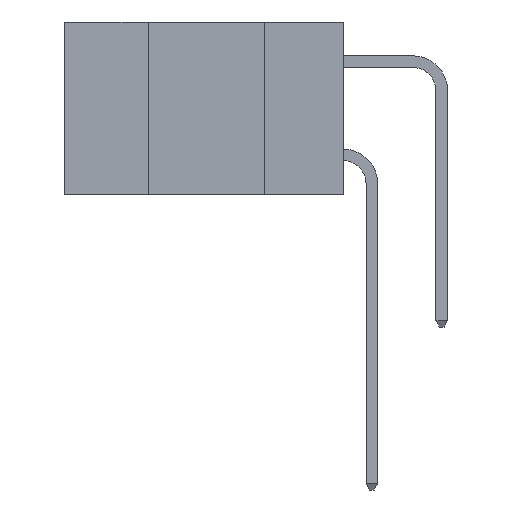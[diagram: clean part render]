
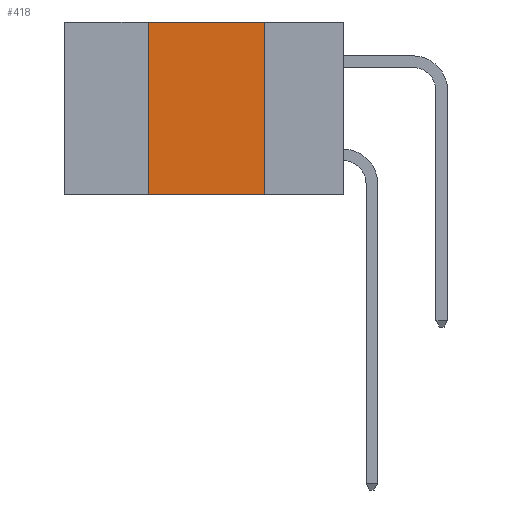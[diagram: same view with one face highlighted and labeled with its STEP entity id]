
A CAD part, left-side view. The second image highlights one B-rep face of the part: STEP entity #418.
In plain terms, the highlighted planar face has unit normal (-1, 0, 0).
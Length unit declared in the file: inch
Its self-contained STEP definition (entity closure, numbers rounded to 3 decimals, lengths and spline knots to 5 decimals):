
#340 = CARTESIAN_POINT ( 'NONE',  ( 0., 0.6, -0.37 ) ) ;
#369 = EDGE_CURVE ( 'NONE', #6488, #3196, #8208, .T. ) ;
#418 = ADVANCED_FACE ( 'NONE', ( #5641 ), #8332, .F. ) ;
#494 = AXIS2_PLACEMENT_3D ( 'NONE', #7348, #6363, #9915 ) ;
#639 = EDGE_CURVE ( 'NONE', #6488, #5417, #9170, .T. ) ;
#745 = DIRECTION ( 'NONE',  ( 0., -1., 0. ) ) ;
#939 = CARTESIAN_POINT ( 'NONE',  ( 0., 0.6, 0. ) ) ;
#1152 = VERTEX_POINT ( 'NONE', #2758 ) ;
#2500 = VECTOR ( 'NONE', #10868, 39.37008 ) ;
#2507 = ORIENTED_EDGE ( 'NONE', *, *, #369, .T. ) ;
#2758 = CARTESIAN_POINT ( 'NONE',  ( 0., 0.17, 0. ) ) ;
#3020 = LINE ( 'NONE', #939, #2500 ) ;
#3196 = VERTEX_POINT ( 'NONE', #7700 ) ;
#3681 = CARTESIAN_POINT ( 'NONE',  ( 0., 0.42, -0.37 ) ) ;
#3735 = DIRECTION ( 'NONE',  ( 0., 0., 1. ) ) ;
#4081 = CARTESIAN_POINT ( 'NONE',  ( 0., 0.42, 0. ) ) ;
#4154 = EDGE_CURVE ( 'NONE', #5417, #1152, #3020, .T. ) ;
#4572 = EDGE_CURVE ( 'NONE', #1152, #3196, #6546, .T. ) ;
#4858 = VECTOR ( 'NONE', #3735, 39.37008 ) ;
#4903 = DIRECTION ( 'NONE',  ( 0., 0., -1. ) ) ;
#5268 = VECTOR ( 'NONE', #745, 39.37008 ) ;
#5321 = ORIENTED_EDGE ( 'NONE', *, *, #4572, .F. ) ;
#5417 = VERTEX_POINT ( 'NONE', #4081 ) ;
#5641 = FACE_OUTER_BOUND ( 'NONE', #7751, .T. ) ;
#6363 = DIRECTION ( 'NONE',  ( 1., 0., 0. ) ) ;
#6488 = VERTEX_POINT ( 'NONE', #10600 ) ;
#6546 = LINE ( 'NONE', #10422, #8708 ) ;
#6943 = ORIENTED_EDGE ( 'NONE', *, *, #4154, .F. ) ;
#7348 = CARTESIAN_POINT ( 'NONE',  ( 0., 0.6, 0. ) ) ;
#7700 = CARTESIAN_POINT ( 'NONE',  ( 0., 0.17, -0.37 ) ) ;
#7751 = EDGE_LOOP ( 'NONE', ( #5321, #6943, #9878, #2507 ) ) ;
#8208 = LINE ( 'NONE', #340, #5268 ) ;
#8332 = PLANE ( 'NONE',  #494 ) ;
#8708 = VECTOR ( 'NONE', #4903, 39.37008 ) ;
#9170 = LINE ( 'NONE', #3681, #4858 ) ;
#9878 = ORIENTED_EDGE ( 'NONE', *, *, #639, .F. ) ;
#9915 = DIRECTION ( 'NONE',  ( 0., 0., -1. ) ) ;
#10422 = CARTESIAN_POINT ( 'NONE',  ( 0., 0.17, -0.37 ) ) ;
#10600 = CARTESIAN_POINT ( 'NONE',  ( 0., 0.42, -0.37 ) ) ;
#10868 = DIRECTION ( 'NONE',  ( 0., -1., 0. ) ) ;
